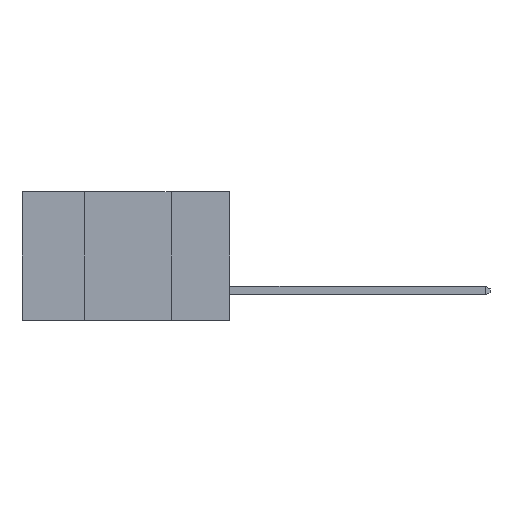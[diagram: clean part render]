
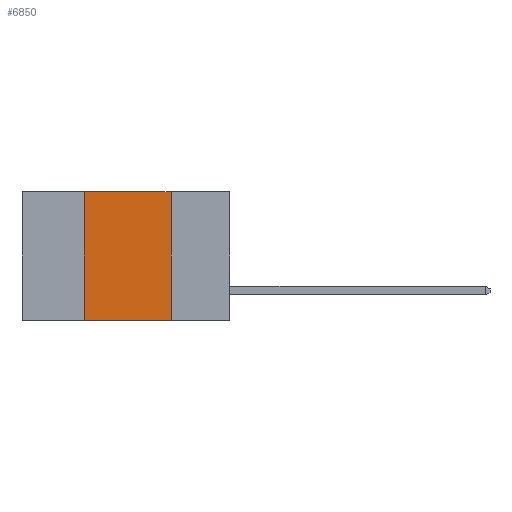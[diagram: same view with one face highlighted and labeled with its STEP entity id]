
A CAD part, left-side view. The second image highlights one B-rep face of the part: STEP entity #6850.
In plain terms, the highlighted planar face has unit normal (-1, 0, 0).
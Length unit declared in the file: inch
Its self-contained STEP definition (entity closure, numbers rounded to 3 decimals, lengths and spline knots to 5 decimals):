
#550 = CARTESIAN_POINT ( 'NONE',  ( 0., 0.42, 0. ) ) ;
#553 = ORIENTED_EDGE ( 'NONE', *, *, #6999, .T. ) ;
#1291 = PLANE ( 'NONE',  #7255 ) ;
#1829 = DIRECTION ( 'NONE',  ( 0., 0., 1. ) ) ;
#2007 = CARTESIAN_POINT ( 'NONE',  ( 0., 0.17, -0.37 ) ) ;
#2581 = DIRECTION ( 'NONE',  ( 0., 0., -1. ) ) ;
#2879 = CARTESIAN_POINT ( 'NONE',  ( 0., 0.6, -0.37 ) ) ;
#3192 = ORIENTED_EDGE ( 'NONE', *, *, #8750, .F. ) ;
#3616 = ORIENTED_EDGE ( 'NONE', *, *, #15159, .F. ) ;
#4088 = CARTESIAN_POINT ( 'NONE',  ( 0., 0.17, 0. ) ) ;
#4643 = VECTOR ( 'NONE', #12655, 39.37008 ) ;
#5000 = LINE ( 'NONE', #4088, #14402 ) ;
#6179 = VECTOR ( 'NONE', #15085, 39.37008 ) ;
#6307 = CARTESIAN_POINT ( 'NONE',  ( 0., 0.42, 0. ) ) ;
#6850 = ADVANCED_FACE ( 'NONE', ( #10052 ), #1291, .F. ) ;
#6885 = CARTESIAN_POINT ( 'NONE',  ( 0., 0.6, 0. ) ) ;
#6999 = EDGE_CURVE ( 'NONE', #9547, #7201, #14084, .T. ) ;
#7201 = VERTEX_POINT ( 'NONE', #2007 ) ;
#7255 = AXIS2_PLACEMENT_3D ( 'NONE', #13515, #9982, #2581 ) ;
#8121 = CARTESIAN_POINT ( 'NONE',  ( 0., 0.42, -0.37 ) ) ;
#8750 = EDGE_CURVE ( 'NONE', #9474, #7201, #5000, .T. ) ;
#8786 = VECTOR ( 'NONE', #1829, 39.37008 ) ;
#9474 = VERTEX_POINT ( 'NONE', #11501 ) ;
#9547 = VERTEX_POINT ( 'NONE', #8121 ) ;
#9982 = DIRECTION ( 'NONE',  ( 1., 0., 0. ) ) ;
#10052 = FACE_OUTER_BOUND ( 'NONE', #14045, .T. ) ;
#10085 = ORIENTED_EDGE ( 'NONE', *, *, #14550, .F. ) ;
#11305 = DIRECTION ( 'NONE',  ( 0., 0., -1. ) ) ;
#11501 = CARTESIAN_POINT ( 'NONE',  ( 0., 0.17, 0. ) ) ;
#12655 = DIRECTION ( 'NONE',  ( 0., -1., 0. ) ) ;
#13515 = CARTESIAN_POINT ( 'NONE',  ( 0., 0.6, 0. ) ) ;
#14045 = EDGE_LOOP ( 'NONE', ( #3192, #3616, #10085, #553 ) ) ;
#14084 = LINE ( 'NONE', #2879, #4643 ) ;
#14255 = VERTEX_POINT ( 'NONE', #6307 ) ;
#14402 = VECTOR ( 'NONE', #11305, 39.37008 ) ;
#14550 = EDGE_CURVE ( 'NONE', #9547, #14255, #14668, .T. ) ;
#14668 = LINE ( 'NONE', #550, #8786 ) ;
#14836 = LINE ( 'NONE', #6885, #6179 ) ;
#15085 = DIRECTION ( 'NONE',  ( 0., -1., 0. ) ) ;
#15159 = EDGE_CURVE ( 'NONE', #14255, #9474, #14836, .T. ) ;
